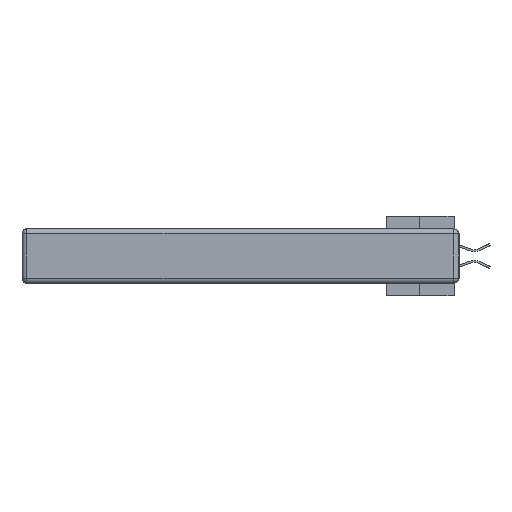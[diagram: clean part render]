
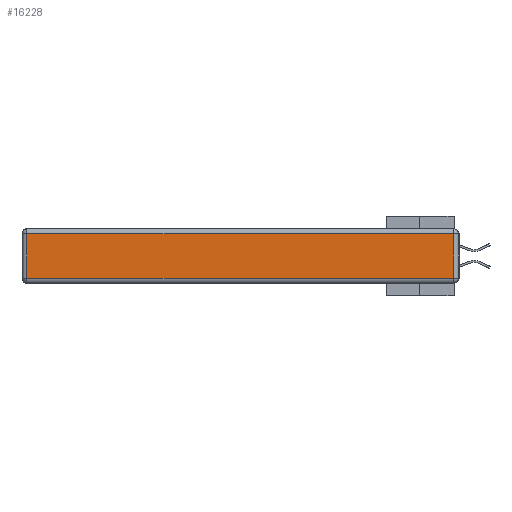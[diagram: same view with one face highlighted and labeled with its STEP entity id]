
A CAD part, left-side view. The second image highlights one B-rep face of the part: STEP entity #16228.
In plain terms, the highlighted planar face has unit normal (-1, 0, 0).
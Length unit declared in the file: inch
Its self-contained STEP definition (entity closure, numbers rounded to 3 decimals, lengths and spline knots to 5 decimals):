
#2055 = EDGE_LOOP ( 'NONE', ( #7543, #2496, #22680, #28224 ) ) ;
#2496 = ORIENTED_EDGE ( 'NONE', *, *, #26409, .T. ) ;
#4314 = CARTESIAN_POINT ( 'NONE',  ( 0., 2.75, -0.03 ) ) ;
#5662 = VERTEX_POINT ( 'NONE', #26797 ) ;
#7447 = DIRECTION ( 'NONE',  ( -1., 0., 0. ) ) ;
#7543 = ORIENTED_EDGE ( 'NONE', *, *, #15584, .T. ) ;
#7804 = LINE ( 'NONE', #19564, #7893 ) ;
#7893 = VECTOR ( 'NONE', #31951, 39.37008 ) ;
#8434 = FACE_OUTER_BOUND ( 'NONE', #2055, .T. ) ;
#9567 = VECTOR ( 'NONE', #16985, 39.37008 ) ;
#9952 = VERTEX_POINT ( 'NONE', #27402 ) ;
#10889 = CARTESIAN_POINT ( 'NONE',  ( 0., 2.72, -0.343 ) ) ;
#12815 = VECTOR ( 'NONE', #18723, 39.37008 ) ;
#13737 = EDGE_CURVE ( 'NONE', #9952, #5662, #32889, .T. ) ;
#13939 = LINE ( 'NONE', #32322, #25827 ) ;
#15584 = EDGE_CURVE ( 'NONE', #5662, #22577, #13939, .T. ) ;
#16097 = CARTESIAN_POINT ( 'NONE',  ( 0., 0., -0.343 ) ) ;
#16228 = ADVANCED_FACE ( 'NONE', ( #8434 ), #33865, .T. ) ;
#16985 = DIRECTION ( 'NONE',  ( 0., 0., -1. ) ) ;
#17320 = LINE ( 'NONE', #4314, #12815 ) ;
#18421 = AXIS2_PLACEMENT_3D ( 'NONE', #16097, #7447, #34120 ) ;
#18465 = CARTESIAN_POINT ( 'NONE',  ( 0., 0.03, -0.313 ) ) ;
#18723 = DIRECTION ( 'NONE',  ( 0., 1., 0. ) ) ;
#19564 = CARTESIAN_POINT ( 'NONE',  ( 0., 0.03, -0.343 ) ) ;
#22577 = VERTEX_POINT ( 'NONE', #18465 ) ;
#22680 = ORIENTED_EDGE ( 'NONE', *, *, #36661, .T. ) ;
#25827 = VECTOR ( 'NONE', #26576, 39.37008 ) ;
#26093 = VERTEX_POINT ( 'NONE', #27139 ) ;
#26409 = EDGE_CURVE ( 'NONE', #22577, #26093, #7804, .T. ) ;
#26576 = DIRECTION ( 'NONE',  ( 0., -1., 0. ) ) ;
#26797 = CARTESIAN_POINT ( 'NONE',  ( 0., 2.72, -0.313 ) ) ;
#27139 = CARTESIAN_POINT ( 'NONE',  ( 0., 0.03, -0.03 ) ) ;
#27402 = CARTESIAN_POINT ( 'NONE',  ( 0., 2.72, -0.03 ) ) ;
#28224 = ORIENTED_EDGE ( 'NONE', *, *, #13737, .T. ) ;
#31951 = DIRECTION ( 'NONE',  ( 0., 0., 1. ) ) ;
#32322 = CARTESIAN_POINT ( 'NONE',  ( 0., 0., -0.313 ) ) ;
#32889 = LINE ( 'NONE', #10889, #9567 ) ;
#33865 = PLANE ( 'NONE',  #18421 ) ;
#34120 = DIRECTION ( 'NONE',  ( 0., 0., 1. ) ) ;
#36661 = EDGE_CURVE ( 'NONE', #26093, #9952, #17320, .T. ) ;
